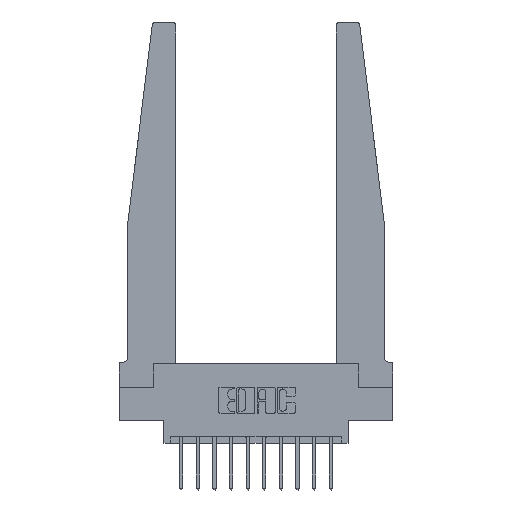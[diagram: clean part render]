
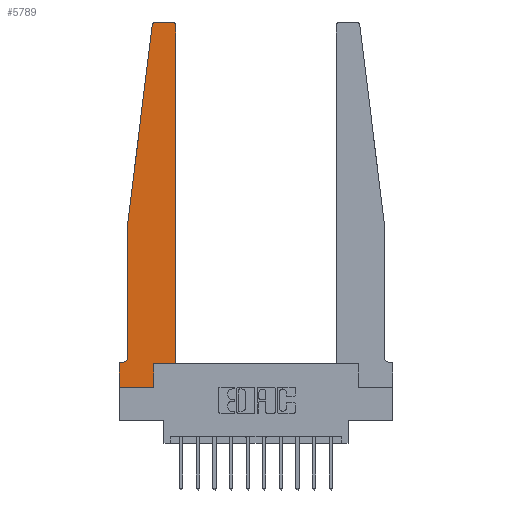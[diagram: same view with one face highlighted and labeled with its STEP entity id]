
A CAD part, top view. The second image highlights one B-rep face of the part: STEP entity #5789.
In plain terms, the highlighted planar face has unit normal (0, 0, 1).
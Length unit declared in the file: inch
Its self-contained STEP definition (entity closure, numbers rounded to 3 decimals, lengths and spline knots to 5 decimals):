
#108 = CIRCLE ( 'NONE', #1948, 0.03 ) ;
#236 = VECTOR ( 'NONE', #5026, 39.37008 ) ;
#305 = CIRCLE ( 'NONE', #13656, 0.05 ) ;
#317 = DIRECTION ( 'NONE',  ( 0., -1., 0. ) ) ;
#378 = AXIS2_PLACEMENT_3D ( 'NONE', #9807, #11048, #2172 ) ;
#406 = CARTESIAN_POINT ( 'NONE',  ( 0.065, 0.1875, 0.37 ) ) ;
#413 = EDGE_CURVE ( 'NONE', #8143, #12792, #108, .T. ) ;
#436 = CARTESIAN_POINT ( 'NONE',  ( 0.2605, 0.18, 0.37 ) ) ;
#609 = VECTOR ( 'NONE', #12861, 39.37008 ) ;
#748 = ORIENTED_EDGE ( 'NONE', *, *, #15497, .T. ) ;
#827 = DIRECTION ( 'NONE',  ( 0., 1., 0. ) ) ;
#1073 = CARTESIAN_POINT ( 'NONE',  ( 0.24675, 2.72367, 0.37 ) ) ;
#1089 = VECTOR ( 'NONE', #1765, 39.37008 ) ;
#1252 = DIRECTION ( 'NONE',  ( 1., 0., 0. ) ) ;
#1376 = DIRECTION ( 'NONE',  ( -1., 0., 0. ) ) ;
#1555 = ORIENTED_EDGE ( 'NONE', *, *, #14125, .T. ) ;
#1659 = VERTEX_POINT ( 'NONE', #8721 ) ;
#1765 = DIRECTION ( 'NONE',  ( 1., 0., 0. ) ) ;
#1948 = AXIS2_PLACEMENT_3D ( 'NONE', #10244, #2706, #7730 ) ;
#2051 = LINE ( 'NONE', #12067, #3143 ) ;
#2054 = DIRECTION ( 'NONE',  ( -0.122, -0.992, 0. ) ) ;
#2080 = VERTEX_POINT ( 'NONE', #2857 ) ;
#2172 = DIRECTION ( 'NONE',  ( 1., 0., 0. ) ) ;
#2309 = CARTESIAN_POINT ( 'NONE',  ( 0.425, 0.18, 0.37 ) ) ;
#2346 = VERTEX_POINT ( 'NONE', #12188 ) ;
#2706 = DIRECTION ( 'NONE',  ( 0., 0., 1. ) ) ;
#2857 = CARTESIAN_POINT ( 'NONE',  ( 0., 0., 0.37 ) ) ;
#2946 = VECTOR ( 'NONE', #4101, 39.37008 ) ;
#3143 = VECTOR ( 'NONE', #827, 39.37008 ) ;
#3456 = VERTEX_POINT ( 'NONE', #2309 ) ;
#3469 = EDGE_CURVE ( 'NONE', #2346, #4810, #6178, .T. ) ;
#3703 = VERTEX_POINT ( 'NONE', #10254 ) ;
#3842 = ORIENTED_EDGE ( 'NONE', *, *, #11154, .T. ) ;
#3982 = ORIENTED_EDGE ( 'NONE', *, *, #3469, .T. ) ;
#4101 = DIRECTION ( 'NONE',  ( 0., -1., 0. ) ) ;
#4130 = CARTESIAN_POINT ( 'NONE',  ( 0.425, 0.18, 0.37 ) ) ;
#4422 = VERTEX_POINT ( 'NONE', #14525 ) ;
#4810 = VERTEX_POINT ( 'NONE', #12828 ) ;
#4989 = DIRECTION ( 'NONE',  ( 0., 0., -1. ) ) ;
#5026 = DIRECTION ( 'NONE',  ( -1., 0., 0. ) ) ;
#5141 = CARTESIAN_POINT ( 'NONE',  ( 0., 0.1875, 0.37 ) ) ;
#5153 = EDGE_CURVE ( 'NONE', #12792, #4422, #13303, .T. ) ;
#5411 = ORIENTED_EDGE ( 'NONE', *, *, #12724, .T. ) ;
#5471 = CARTESIAN_POINT ( 'NONE',  ( 0.27653, 2.75, 0.37 ) ) ;
#5639 = VECTOR ( 'NONE', #8802, 39.37008 ) ;
#5789 = ADVANCED_FACE ( 'NONE', ( #13635 ), #8405, .T. ) ;
#5838 = CARTESIAN_POINT ( 'NONE',  ( 0.065, 1.25, 0.37 ) ) ;
#6178 = CIRCLE ( 'NONE', #15329, 0.03 ) ;
#6384 = CARTESIAN_POINT ( 'NONE',  ( 0.015, 0.2375, 0.37 ) ) ;
#6420 = VECTOR ( 'NONE', #317, 39.37008 ) ;
#6635 = ORIENTED_EDGE ( 'NONE', *, *, #13458, .T. ) ;
#6800 = CARTESIAN_POINT ( 'NONE',  ( 0., 0., 0.37 ) ) ;
#7197 = VERTEX_POINT ( 'NONE', #436 ) ;
#7730 = DIRECTION ( 'NONE',  ( 1., 0., 0. ) ) ;
#7749 = LINE ( 'NONE', #12735, #6420 ) ;
#7809 = VERTEX_POINT ( 'NONE', #14167 ) ;
#8143 = VERTEX_POINT ( 'NONE', #5471 ) ;
#8405 = PLANE ( 'NONE',  #378 ) ;
#8576 = EDGE_CURVE ( 'NONE', #1659, #7197, #9095, .T. ) ;
#8721 = CARTESIAN_POINT ( 'NONE',  ( 0.2605, 0., 0.37 ) ) ;
#8802 = DIRECTION ( 'NONE',  ( -1., 0., 0. ) ) ;
#8834 = ORIENTED_EDGE ( 'NONE', *, *, #5153, .T. ) ;
#9095 = LINE ( 'NONE', #11613, #609 ) ;
#9807 = CARTESIAN_POINT ( 'NONE',  ( 0., 0.1875, 0.37 ) ) ;
#9921 = ORIENTED_EDGE ( 'NONE', *, *, #13802, .T. ) ;
#10008 = LINE ( 'NONE', #6800, #2946 ) ;
#10197 = LINE ( 'NONE', #4130, #15658 ) ;
#10244 = CARTESIAN_POINT ( 'NONE',  ( 0.27653, 2.72, 0.37 ) ) ;
#10254 = CARTESIAN_POINT ( 'NONE',  ( 0.015, 0.1875, 0.37 ) ) ;
#10635 = CARTESIAN_POINT ( 'NONE',  ( 0., 0., 0.37 ) ) ;
#11026 = ORIENTED_EDGE ( 'NONE', *, *, #413, .T. ) ;
#11048 = DIRECTION ( 'NONE',  ( 0., 0., 1. ) ) ;
#11136 = VECTOR ( 'NONE', #2054, 39.37008 ) ;
#11154 = EDGE_CURVE ( 'NONE', #7197, #3456, #10197, .T. ) ;
#11493 = DIRECTION ( 'NONE',  ( 1., 0., 0. ) ) ;
#11521 = LINE ( 'NONE', #10635, #1089 ) ;
#11613 = CARTESIAN_POINT ( 'NONE',  ( 0.2605, 0.18, 0.37 ) ) ;
#11720 = ORIENTED_EDGE ( 'NONE', *, *, #8576, .T. ) ;
#12067 = CARTESIAN_POINT ( 'NONE',  ( 0.425, 0.18, 0.37 ) ) ;
#12188 = CARTESIAN_POINT ( 'NONE',  ( 0.425, 2.72, 0.37 ) ) ;
#12317 = EDGE_CURVE ( 'NONE', #4810, #8143, #14675, .T. ) ;
#12724 = EDGE_CURVE ( 'NONE', #3456, #2346, #2051, .T. ) ;
#12735 = CARTESIAN_POINT ( 'NONE',  ( 0.065, 1.25, 0.37 ) ) ;
#12792 = VERTEX_POINT ( 'NONE', #1073 ) ;
#12828 = CARTESIAN_POINT ( 'NONE',  ( 0.395, 2.75, 0.37 ) ) ;
#12861 = DIRECTION ( 'NONE',  ( 0., 1., 0. ) ) ;
#12897 = ORIENTED_EDGE ( 'NONE', *, *, #12317, .T. ) ;
#12947 = ORIENTED_EDGE ( 'NONE', *, *, #14102, .T. ) ;
#13303 = LINE ( 'NONE', #5838, #11136 ) ;
#13458 = EDGE_CURVE ( 'NONE', #13689, #2080, #10008, .T. ) ;
#13550 = CARTESIAN_POINT ( 'NONE',  ( 0.25, 2.75, 0.37 ) ) ;
#13606 = DIRECTION ( 'NONE',  ( 0., 0., 1. ) ) ;
#13635 = FACE_OUTER_BOUND ( 'NONE', #14301, .T. ) ;
#13656 = AXIS2_PLACEMENT_3D ( 'NONE', #6384, #4989, #1376 ) ;
#13689 = VERTEX_POINT ( 'NONE', #5141 ) ;
#13802 = EDGE_CURVE ( 'NONE', #2080, #1659, #11521, .T. ) ;
#14081 = LINE ( 'NONE', #406, #5639 ) ;
#14102 = EDGE_CURVE ( 'NONE', #4422, #7809, #7749, .T. ) ;
#14125 = EDGE_CURVE ( 'NONE', #3703, #13689, #14081, .T. ) ;
#14167 = CARTESIAN_POINT ( 'NONE',  ( 0.065, 0.2375, 0.37 ) ) ;
#14301 = EDGE_LOOP ( 'NONE', ( #12897, #11026, #8834, #12947, #748, #1555, #6635, #9921, #11720, #3842, #5411, #3982 ) ) ;
#14525 = CARTESIAN_POINT ( 'NONE',  ( 0.065, 1.25, 0.37 ) ) ;
#14675 = LINE ( 'NONE', #13550, #236 ) ;
#14755 = CARTESIAN_POINT ( 'NONE',  ( 0.395, 2.72, 0.37 ) ) ;
#15329 = AXIS2_PLACEMENT_3D ( 'NONE', #14755, #13606, #1252 ) ;
#15497 = EDGE_CURVE ( 'NONE', #7809, #3703, #305, .T. ) ;
#15658 = VECTOR ( 'NONE', #11493, 39.37008 ) ;
